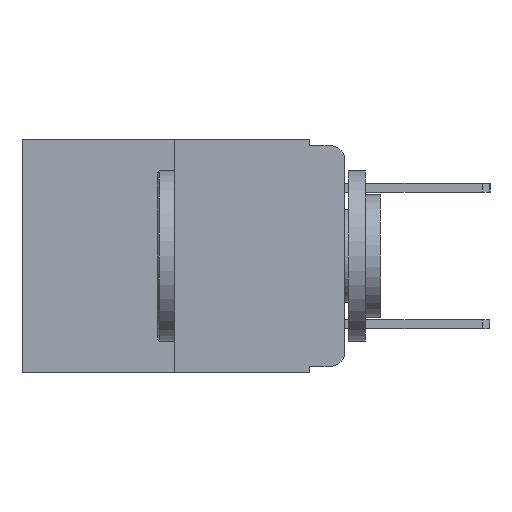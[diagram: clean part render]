
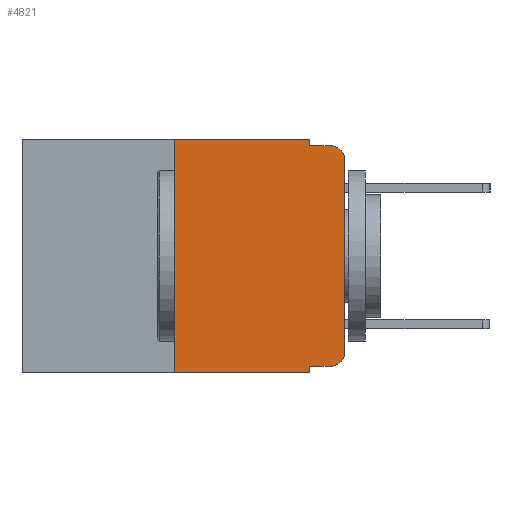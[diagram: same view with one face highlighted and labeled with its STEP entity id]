
A CAD part, left-side view. The second image highlights one B-rep face of the part: STEP entity #4821.
In plain terms, the highlighted planar face has unit normal (-1, 0, 0).
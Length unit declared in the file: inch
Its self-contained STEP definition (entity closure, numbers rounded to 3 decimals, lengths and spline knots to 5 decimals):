
#70 = VERTEX_POINT ( 'NONE', #8578 ) ;
#113 = EDGE_CURVE ( 'NONE', #4801, #11277, #3480, .T. ) ;
#146 = CARTESIAN_POINT ( 'NONE',  ( 0., 0.02, -0.01 ) ) ;
#240 = VECTOR ( 'NONE', #7785, 39.37008 ) ;
#300 = EDGE_CURVE ( 'NONE', #4003, #4801, #3907, .T. ) ;
#521 = DIRECTION ( 'NONE',  ( 0., 0., 1. ) ) ;
#528 = CARTESIAN_POINT ( 'NONE',  ( 0., 0., -0.03 ) ) ;
#567 = CARTESIAN_POINT ( 'NONE',  ( 0., 0.02, -0.03 ) ) ;
#874 = LINE ( 'NONE', #4156, #10359 ) ;
#1000 = ORIENTED_EDGE ( 'NONE', *, *, #9730, .F. ) ;
#1034 = CARTESIAN_POINT ( 'NONE',  ( 0., 0.25, 0. ) ) ;
#1080 = VERTEX_POINT ( 'NONE', #5513 ) ;
#1406 = AXIS2_PLACEMENT_3D ( 'NONE', #9470, #4062, #2664 ) ;
#1600 = DIRECTION ( 'NONE',  ( 0., 0., -1. ) ) ;
#1696 = DIRECTION ( 'NONE',  ( 0., 0., -1. ) ) ;
#1755 = VERTEX_POINT ( 'NONE', #9356 ) ;
#1900 = VECTOR ( 'NONE', #5830, 39.37008 ) ;
#1915 = CARTESIAN_POINT ( 'NONE',  ( 0., 0.051, -0.333 ) ) ;
#2257 = ORIENTED_EDGE ( 'NONE', *, *, #8873, .T. ) ;
#2525 = DIRECTION ( 'NONE',  ( 0., -1., 0. ) ) ;
#2556 = LINE ( 'NONE', #10141, #12118 ) ;
#2664 = DIRECTION ( 'NONE',  ( 0., 0., -1. ) ) ;
#2678 = CARTESIAN_POINT ( 'NONE',  ( 0., 0.051, -0.333 ) ) ;
#2908 = CARTESIAN_POINT ( 'NONE',  ( 0., 0.473, 0. ) ) ;
#3019 = EDGE_CURVE ( 'NONE', #11810, #4003, #4861, .T. ) ;
#3352 = DIRECTION ( 'NONE',  ( 0., -1., 0. ) ) ;
#3480 = LINE ( 'NONE', #11627, #8820 ) ;
#3907 = CIRCLE ( 'NONE', #1406, 0.02 ) ;
#4003 = VERTEX_POINT ( 'NONE', #5919 ) ;
#4057 = DIRECTION ( 'NONE',  ( 0., -1., 0. ) ) ;
#4062 = DIRECTION ( 'NONE',  ( -1., 0., 0. ) ) ;
#4156 = CARTESIAN_POINT ( 'NONE',  ( 0., 0.473, -0.343 ) ) ;
#4244 = EDGE_CURVE ( 'NONE', #70, #6623, #9655, .T. ) ;
#4257 = VECTOR ( 'NONE', #2525, 39.37008 ) ;
#4694 = VERTEX_POINT ( 'NONE', #8536 ) ;
#4801 = VERTEX_POINT ( 'NONE', #11755 ) ;
#4821 = ADVANCED_FACE ( 'NONE', ( #11150 ), #11262, .F. ) ;
#4861 = LINE ( 'NONE', #1915, #4257 ) ;
#5513 = CARTESIAN_POINT ( 'NONE',  ( 0., 0.051, -0.343 ) ) ;
#5830 = DIRECTION ( 'NONE',  ( 0., 0., -1. ) ) ;
#5895 = ORIENTED_EDGE ( 'NONE', *, *, #113, .T. ) ;
#5919 = CARTESIAN_POINT ( 'NONE',  ( 0., 0.02, -0.333 ) ) ;
#5939 = ORIENTED_EDGE ( 'NONE', *, *, #9447, .F. ) ;
#5998 = CARTESIAN_POINT ( 'NONE',  ( 0., 0.051, -0.01 ) ) ;
#6142 = ORIENTED_EDGE ( 'NONE', *, *, #6441, .F. ) ;
#6184 = LINE ( 'NONE', #5998, #10766 ) ;
#6441 = EDGE_CURVE ( 'NONE', #6623, #1755, #11811, .T. ) ;
#6623 = VERTEX_POINT ( 'NONE', #10604 ) ;
#7260 = ORIENTED_EDGE ( 'NONE', *, *, #7751, .T. ) ;
#7356 = DIRECTION ( 'NONE',  ( -1., 0., 0. ) ) ;
#7477 = ORIENTED_EDGE ( 'NONE', *, *, #4244, .F. ) ;
#7648 = ORIENTED_EDGE ( 'NONE', *, *, #3019, .T. ) ;
#7751 = EDGE_CURVE ( 'NONE', #11277, #9441, #8051, .T. ) ;
#7785 = DIRECTION ( 'NONE',  ( 0., 0., 1. ) ) ;
#7885 = EDGE_LOOP ( 'NONE', ( #5895, #7260, #5939, #6142, #7477, #10156, #2257, #1000, #7648, #11612 ) ) ;
#7973 = AXIS2_PLACEMENT_3D ( 'NONE', #567, #7356, #1600 ) ;
#8051 = CIRCLE ( 'NONE', #7973, 0.02 ) ;
#8419 = AXIS2_PLACEMENT_3D ( 'NONE', #11318, #11180, #11142 ) ;
#8536 = CARTESIAN_POINT ( 'NONE',  ( 0., 0.25, -0.343 ) ) ;
#8578 = CARTESIAN_POINT ( 'NONE',  ( 0., 0.25, 0. ) ) ;
#8820 = VECTOR ( 'NONE', #521, 39.37008 ) ;
#8873 = EDGE_CURVE ( 'NONE', #4694, #1080, #874, .T. ) ;
#9356 = CARTESIAN_POINT ( 'NONE',  ( 0., 0.051, -0.01 ) ) ;
#9363 = EDGE_CURVE ( 'NONE', #4694, #70, #11857, .T. ) ;
#9387 = VECTOR ( 'NONE', #3352, 39.37008 ) ;
#9441 = VERTEX_POINT ( 'NONE', #146 ) ;
#9447 = EDGE_CURVE ( 'NONE', #1755, #9441, #6184, .T. ) ;
#9470 = CARTESIAN_POINT ( 'NONE',  ( 0., 0.02, -0.313 ) ) ;
#9655 = LINE ( 'NONE', #2908, #9387 ) ;
#9730 = EDGE_CURVE ( 'NONE', #11810, #1080, #2556, .T. ) ;
#10141 = CARTESIAN_POINT ( 'NONE',  ( 0., 0.051, 0. ) ) ;
#10156 = ORIENTED_EDGE ( 'NONE', *, *, #9363, .F. ) ;
#10359 = VECTOR ( 'NONE', #11534, 39.37008 ) ;
#10410 = CARTESIAN_POINT ( 'NONE',  ( 0., 0.051, 0. ) ) ;
#10604 = CARTESIAN_POINT ( 'NONE',  ( 0., 0.051, 0. ) ) ;
#10766 = VECTOR ( 'NONE', #4057, 39.37008 ) ;
#11142 = DIRECTION ( 'NONE',  ( 0., 0., -1. ) ) ;
#11150 = FACE_OUTER_BOUND ( 'NONE', #7885, .T. ) ;
#11180 = DIRECTION ( 'NONE',  ( 1., 0., 0. ) ) ;
#11262 = PLANE ( 'NONE',  #8419 ) ;
#11277 = VERTEX_POINT ( 'NONE', #528 ) ;
#11318 = CARTESIAN_POINT ( 'NONE',  ( 0., 0.473, 0. ) ) ;
#11534 = DIRECTION ( 'NONE',  ( 0., -1., 0. ) ) ;
#11612 = ORIENTED_EDGE ( 'NONE', *, *, #300, .T. ) ;
#11627 = CARTESIAN_POINT ( 'NONE',  ( 0., 0., 0. ) ) ;
#11755 = CARTESIAN_POINT ( 'NONE',  ( 0., 0., -0.313 ) ) ;
#11810 = VERTEX_POINT ( 'NONE', #2678 ) ;
#11811 = LINE ( 'NONE', #10410, #1900 ) ;
#11857 = LINE ( 'NONE', #1034, #240 ) ;
#12118 = VECTOR ( 'NONE', #1696, 39.37008 ) ;
